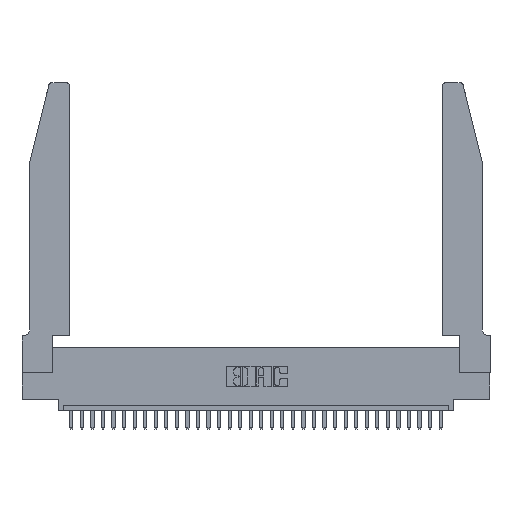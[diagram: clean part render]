
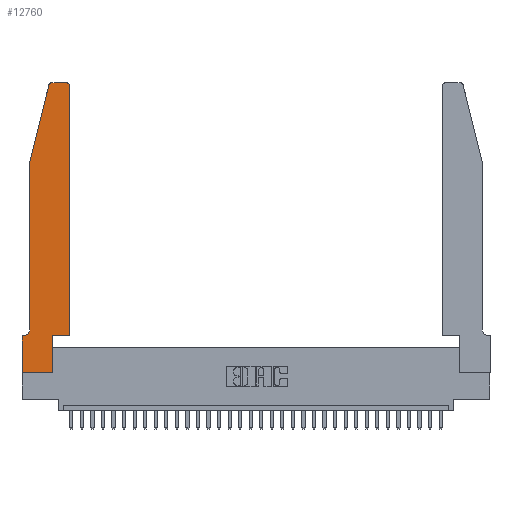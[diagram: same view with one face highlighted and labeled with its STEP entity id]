
A CAD part, top view. The second image highlights one B-rep face of the part: STEP entity #12760.
In plain terms, the highlighted planar face has unit normal (0, 0, 1).
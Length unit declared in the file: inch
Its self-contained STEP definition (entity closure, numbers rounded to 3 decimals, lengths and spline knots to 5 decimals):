
#218 = AXIS2_PLACEMENT_3D ( 'NONE', #4908, #22670, #25199 ) ;
#665 = CIRCLE ( 'NONE', #218, 0.07 ) ;
#693 = CARTESIAN_POINT ( 'NONE',  ( 0.25487, 2.72718, 0.37 ) ) ;
#1235 = AXIS2_PLACEMENT_3D ( 'NONE', #29959, #4924, #28857 ) ;
#1738 = VECTOR ( 'NONE', #6809, 39.37008 ) ;
#2615 = CARTESIAN_POINT ( 'NONE',  ( 0.4205, 2.75, 0.37 ) ) ;
#4415 = ORIENTED_EDGE ( 'NONE', *, *, #28341, .T. ) ;
#4738 = CARTESIAN_POINT ( 'NONE',  ( 0., 0., 0.37 ) ) ;
#4908 = CARTESIAN_POINT ( 'NONE',  ( 0.0055, 0.42, 0.37 ) ) ;
#4924 = DIRECTION ( 'NONE',  ( 0., 0., 1. ) ) ;
#4978 = VECTOR ( 'NONE', #19304, 39.37008 ) ;
#5396 = CARTESIAN_POINT ( 'NONE',  ( 0.0755, 0.35, 0.37 ) ) ;
#5452 = EDGE_CURVE ( 'NONE', #22866, #24603, #28369, .T. ) ;
#6605 = LINE ( 'NONE', #11259, #12545 ) ;
#6809 = DIRECTION ( 'NONE',  ( 0., -1., 0. ) ) ;
#7002 = CARTESIAN_POINT ( 'NONE',  ( 0.2865, 0., 0.37 ) ) ;
#7752 = VERTEX_POINT ( 'NONE', #23857 ) ;
#7929 = CARTESIAN_POINT ( 'NONE',  ( 0.4205, 2.72, 0.37 ) ) ;
#8070 = CARTESIAN_POINT ( 'NONE',  ( 0.0755, 2., 0.37 ) ) ;
#8350 = ORIENTED_EDGE ( 'NONE', *, *, #19502, .T. ) ;
#8796 = CARTESIAN_POINT ( 'NONE',  ( 0.4505, 2.72, 0.37 ) ) ;
#9047 = ORIENTED_EDGE ( 'NONE', *, *, #25133, .T. ) ;
#9483 = VERTEX_POINT ( 'NONE', #27535 ) ;
#9554 = EDGE_CURVE ( 'NONE', #24603, #14244, #28666, .T. ) ;
#9782 = VECTOR ( 'NONE', #32036, 39.37008 ) ;
#11259 = CARTESIAN_POINT ( 'NONE',  ( 0.2865, 0.35, 0.37 ) ) ;
#11262 = ORIENTED_EDGE ( 'NONE', *, *, #23026, .T. ) ;
#11701 = LINE ( 'NONE', #15584, #19616 ) ;
#12545 = VECTOR ( 'NONE', #29398, 39.37008 ) ;
#12760 = ADVANCED_FACE ( 'NONE', ( #18972 ), #21836, .T. ) ;
#13155 = DIRECTION ( 'NONE',  ( -1., 0., 0. ) ) ;
#13607 = CARTESIAN_POINT ( 'NONE',  ( 0., 0.35, 0.37 ) ) ;
#13680 = EDGE_CURVE ( 'NONE', #7752, #31206, #25828, .T. ) ;
#13927 = ORIENTED_EDGE ( 'NONE', *, *, #31188, .T. ) ;
#14244 = VERTEX_POINT ( 'NONE', #2615 ) ;
#14432 = VERTEX_POINT ( 'NONE', #7002 ) ;
#14670 = ORIENTED_EDGE ( 'NONE', *, *, #9554, .T. ) ;
#15100 = ORIENTED_EDGE ( 'NONE', *, *, #13680, .T. ) ;
#15584 = CARTESIAN_POINT ( 'NONE',  ( 0.0755, 2., 0.37 ) ) ;
#15644 = EDGE_CURVE ( 'NONE', #16014, #31509, #665, .T. ) ;
#16014 = VERTEX_POINT ( 'NONE', #27187 ) ;
#16183 = CARTESIAN_POINT ( 'NONE',  ( 0.4505, 0.35, 0.37 ) ) ;
#16948 = ORIENTED_EDGE ( 'NONE', *, *, #17968, .T. ) ;
#17968 = EDGE_CURVE ( 'NONE', #20465, #32268, #18450, .T. ) ;
#18450 = LINE ( 'NONE', #28520, #1738 ) ;
#18531 = CARTESIAN_POINT ( 'NONE',  ( 0.4505, 0.35, 0.37 ) ) ;
#18972 = FACE_OUTER_BOUND ( 'NONE', #28706, .T. ) ;
#19246 = CARTESIAN_POINT ( 'NONE',  ( 0.0055, 0.35, 0.37 ) ) ;
#19304 = DIRECTION ( 'NONE',  ( -1., 0., 0. ) ) ;
#19502 = EDGE_CURVE ( 'NONE', #14432, #21184, #6605, .T. ) ;
#19616 = VECTOR ( 'NONE', #28407, 39.37008 ) ;
#19736 = AXIS2_PLACEMENT_3D ( 'NONE', #20715, #23489, #24463 ) ;
#20098 = LINE ( 'NONE', #5396, #24054 ) ;
#20465 = VERTEX_POINT ( 'NONE', #13607 ) ;
#20571 = DIRECTION ( 'NONE',  ( 0., 0., 1. ) ) ;
#20684 = DIRECTION ( 'NONE',  ( 1., 0., 0. ) ) ;
#20715 = CARTESIAN_POINT ( 'NONE',  ( 0., 0.35, 0.37 ) ) ;
#20736 = ORIENTED_EDGE ( 'NONE', *, *, #5452, .T. ) ;
#21184 = VERTEX_POINT ( 'NONE', #23295 ) ;
#21505 = LINE ( 'NONE', #4738, #21926 ) ;
#21618 = CARTESIAN_POINT ( 'NONE',  ( 0.4505, 0.35, 0.37 ) ) ;
#21836 = PLANE ( 'NONE',  #19736 ) ;
#21926 = VECTOR ( 'NONE', #27991, 39.37008 ) ;
#22190 = ORIENTED_EDGE ( 'NONE', *, *, #31092, .T. ) ;
#22331 = CARTESIAN_POINT ( 'NONE',  ( 0., 0., 0.37 ) ) ;
#22670 = DIRECTION ( 'NONE',  ( 0., 0., -1. ) ) ;
#22707 = LINE ( 'NONE', #8070, #26215 ) ;
#22866 = VERTEX_POINT ( 'NONE', #18531 ) ;
#23026 = EDGE_CURVE ( 'NONE', #31509, #20465, #20098, .T. ) ;
#23152 = LINE ( 'NONE', #21618, #32291 ) ;
#23295 = CARTESIAN_POINT ( 'NONE',  ( 0.2865, 0.35, 0.37 ) ) ;
#23489 = DIRECTION ( 'NONE',  ( 0., 0., 1. ) ) ;
#23857 = CARTESIAN_POINT ( 'NONE',  ( 0.284, 2.75, 0.37 ) ) ;
#24054 = VECTOR ( 'NONE', #13155, 39.37008 ) ;
#24463 = DIRECTION ( 'NONE',  ( 1., 0., 0. ) ) ;
#24603 = VERTEX_POINT ( 'NONE', #8796 ) ;
#24840 = LINE ( 'NONE', #32056, #4978 ) ;
#25133 = EDGE_CURVE ( 'NONE', #21184, #22866, #23152, .T. ) ;
#25199 = DIRECTION ( 'NONE',  ( -1., 0., 0. ) ) ;
#25460 = ORIENTED_EDGE ( 'NONE', *, *, #29030, .T. ) ;
#25828 = CIRCLE ( 'NONE', #1235, 0.03 ) ;
#26215 = VECTOR ( 'NONE', #28206, 39.37008 ) ;
#27187 = CARTESIAN_POINT ( 'NONE',  ( 0.0755, 0.42, 0.37 ) ) ;
#27519 = AXIS2_PLACEMENT_3D ( 'NONE', #7929, #20571, #20684 ) ;
#27535 = CARTESIAN_POINT ( 'NONE',  ( 0.0755, 2., 0.37 ) ) ;
#27991 = DIRECTION ( 'NONE',  ( 1., 0., 0. ) ) ;
#28206 = DIRECTION ( 'NONE',  ( -0.239, -0.971, 0. ) ) ;
#28341 = EDGE_CURVE ( 'NONE', #14244, #7752, #24840, .T. ) ;
#28369 = LINE ( 'NONE', #16183, #9782 ) ;
#28407 = DIRECTION ( 'NONE',  ( 0., -1., 0. ) ) ;
#28520 = CARTESIAN_POINT ( 'NONE',  ( 0., 0., 0.37 ) ) ;
#28666 = CIRCLE ( 'NONE', #27519, 0.03 ) ;
#28706 = EDGE_LOOP ( 'NONE', ( #4415, #15100, #13927, #25460, #29700, #11262, #16948, #22190, #8350, #9047, #20736, #14670 ) ) ;
#28857 = DIRECTION ( 'NONE',  ( 1., 0., 0. ) ) ;
#29030 = EDGE_CURVE ( 'NONE', #9483, #16014, #11701, .T. ) ;
#29234 = DIRECTION ( 'NONE',  ( 1., 0., 0. ) ) ;
#29398 = DIRECTION ( 'NONE',  ( 0., 1., 0. ) ) ;
#29700 = ORIENTED_EDGE ( 'NONE', *, *, #15644, .T. ) ;
#29959 = CARTESIAN_POINT ( 'NONE',  ( 0.284, 2.72, 0.37 ) ) ;
#31092 = EDGE_CURVE ( 'NONE', #32268, #14432, #21505, .T. ) ;
#31188 = EDGE_CURVE ( 'NONE', #31206, #9483, #22707, .T. ) ;
#31206 = VERTEX_POINT ( 'NONE', #693 ) ;
#31509 = VERTEX_POINT ( 'NONE', #19246 ) ;
#32036 = DIRECTION ( 'NONE',  ( 0., 1., 0. ) ) ;
#32056 = CARTESIAN_POINT ( 'NONE',  ( 0.2605, 2.75, 0.37 ) ) ;
#32268 = VERTEX_POINT ( 'NONE', #22331 ) ;
#32291 = VECTOR ( 'NONE', #29234, 39.37008 ) ;
